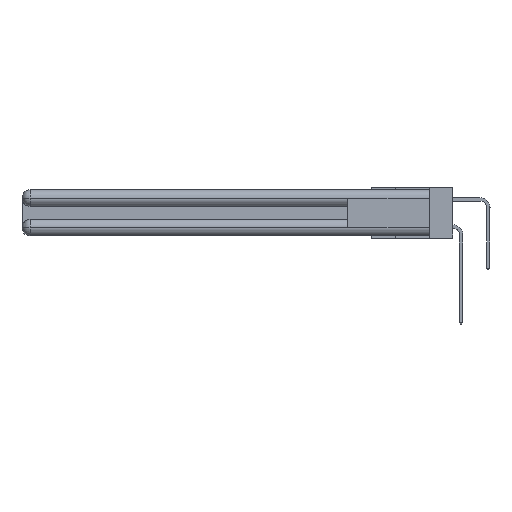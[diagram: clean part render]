
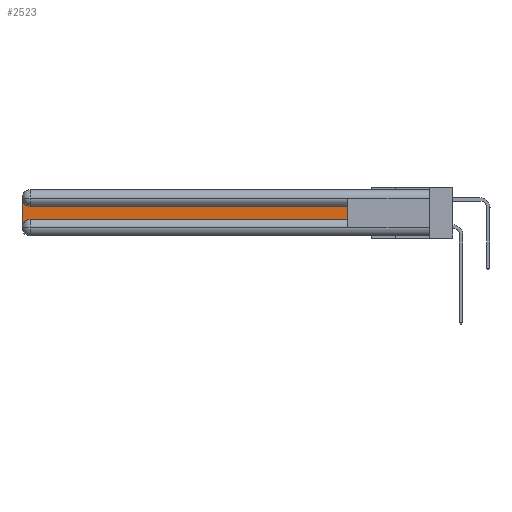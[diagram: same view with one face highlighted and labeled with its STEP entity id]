
A CAD part, left-side view. The second image highlights one B-rep face of the part: STEP entity #2523.
In plain terms, the highlighted planar face has unit normal (-1, 0, 0).
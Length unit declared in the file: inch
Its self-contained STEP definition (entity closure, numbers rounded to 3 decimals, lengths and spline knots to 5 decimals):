
#1633 = AXIS2_PLACEMENT_3D ( 'NONE', #22395, #12397, #30152 ) ;
#1638 = CIRCLE ( 'NONE', #31085, 0.06 ) ;
#1663 = FACE_OUTER_BOUND ( 'NONE', #26943, .T. ) ;
#2435 = EDGE_CURVE ( 'NONE', #10499, #9030, #10544, .T. ) ;
#2523 = ADVANCED_FACE ( 'NONE', ( #1663 ), #9844, .F. ) ;
#3651 = DIRECTION ( 'NONE',  ( 0., 0., 1. ) ) ;
#5877 = EDGE_CURVE ( 'NONE', #27109, #16883, #26396, .T. ) ;
#5898 = DIRECTION ( 'NONE',  ( 0., -1., 0. ) ) ;
#6235 = CARTESIAN_POINT ( 'NONE',  ( 0.075, 0.6, -0.2175 ) ) ;
#7603 = CARTESIAN_POINT ( 'NONE',  ( 0.075, 0.6, -0.2175 ) ) ;
#7732 = VECTOR ( 'NONE', #12460, 39.37008 ) ;
#9030 = VERTEX_POINT ( 'NONE', #14013 ) ;
#9278 = CARTESIAN_POINT ( 'NONE',  ( 0.075, 2.94, -0.2775 ) ) ;
#9844 = PLANE ( 'NONE',  #30306 ) ;
#10313 = CARTESIAN_POINT ( 'NONE',  ( 0.075, 0.6, -0.1225 ) ) ;
#10396 = ORIENTED_EDGE ( 'NONE', *, *, #5877, .T. ) ;
#10499 = VERTEX_POINT ( 'NONE', #30790 ) ;
#10544 = CIRCLE ( 'NONE', #1633, 0.06 ) ;
#10737 = VECTOR ( 'NONE', #5898, 39.37008 ) ;
#10772 = EDGE_CURVE ( 'NONE', #16883, #17466, #19348, .T. ) ;
#10973 = EDGE_CURVE ( 'NONE', #23210, #27109, #1638, .T. ) ;
#11773 = ORIENTED_EDGE ( 'NONE', *, *, #10973, .T. ) ;
#12397 = DIRECTION ( 'NONE',  ( 1., 0., 0. ) ) ;
#12460 = DIRECTION ( 'NONE',  ( 0., 1., 0. ) ) ;
#12582 = VECTOR ( 'NONE', #3651, 39.37008 ) ;
#12584 = LINE ( 'NONE', #10313, #7732 ) ;
#14013 = CARTESIAN_POINT ( 'NONE',  ( 0.075, 3., -0.0625 ) ) ;
#15131 = CARTESIAN_POINT ( 'NONE',  ( 0.075, 3., -0.1225 ) ) ;
#15685 = EDGE_CURVE ( 'NONE', #17466, #10499, #12584, .T. ) ;
#16883 = VERTEX_POINT ( 'NONE', #7603 ) ;
#17466 = VERTEX_POINT ( 'NONE', #23894 ) ;
#17576 = DIRECTION ( 'NONE',  ( 0., 0., -1. ) ) ;
#17925 = EDGE_CURVE ( 'NONE', #9030, #23210, #24419, .T. ) ;
#18461 = ORIENTED_EDGE ( 'NONE', *, *, #15685, .T. ) ;
#19348 = LINE ( 'NONE', #6235, #12582 ) ;
#22395 = CARTESIAN_POINT ( 'NONE',  ( 0.075, 2.94, -0.0625 ) ) ;
#23210 = VERTEX_POINT ( 'NONE', #29079 ) ;
#23745 = ORIENTED_EDGE ( 'NONE', *, *, #17925, .T. ) ;
#23894 = CARTESIAN_POINT ( 'NONE',  ( 0.075, 0.6, -0.1225 ) ) ;
#24419 = LINE ( 'NONE', #27305, #26839 ) ;
#26396 = LINE ( 'NONE', #31183, #10737 ) ;
#26839 = VECTOR ( 'NONE', #29448, 39.37008 ) ;
#26943 = EDGE_LOOP ( 'NONE', ( #18461, #30221, #23745, #11773, #10396, #32229 ) ) ;
#27109 = VERTEX_POINT ( 'NONE', #28774 ) ;
#27305 = CARTESIAN_POINT ( 'NONE',  ( 0.075, 3., -0.2175 ) ) ;
#28147 = DIRECTION ( 'NONE',  ( 1., 0., 0. ) ) ;
#28774 = CARTESIAN_POINT ( 'NONE',  ( 0.075, 2.94, -0.2175 ) ) ;
#29079 = CARTESIAN_POINT ( 'NONE',  ( 0.075, 3., -0.2775 ) ) ;
#29448 = DIRECTION ( 'NONE',  ( 0., 0., -1. ) ) ;
#29618 = DIRECTION ( 'NONE',  ( 1., 0., 0. ) ) ;
#30152 = DIRECTION ( 'NONE',  ( 0., 0., -1. ) ) ;
#30221 = ORIENTED_EDGE ( 'NONE', *, *, #2435, .T. ) ;
#30306 = AXIS2_PLACEMENT_3D ( 'NONE', #15131, #28147, #17576 ) ;
#30790 = CARTESIAN_POINT ( 'NONE',  ( 0.075, 2.94, -0.1225 ) ) ;
#31085 = AXIS2_PLACEMENT_3D ( 'NONE', #9278, #29618, #32401 ) ;
#31183 = CARTESIAN_POINT ( 'NONE',  ( 0.075, 0.6, -0.2175 ) ) ;
#32229 = ORIENTED_EDGE ( 'NONE', *, *, #10772, .T. ) ;
#32401 = DIRECTION ( 'NONE',  ( 0., 0., -1. ) ) ;
